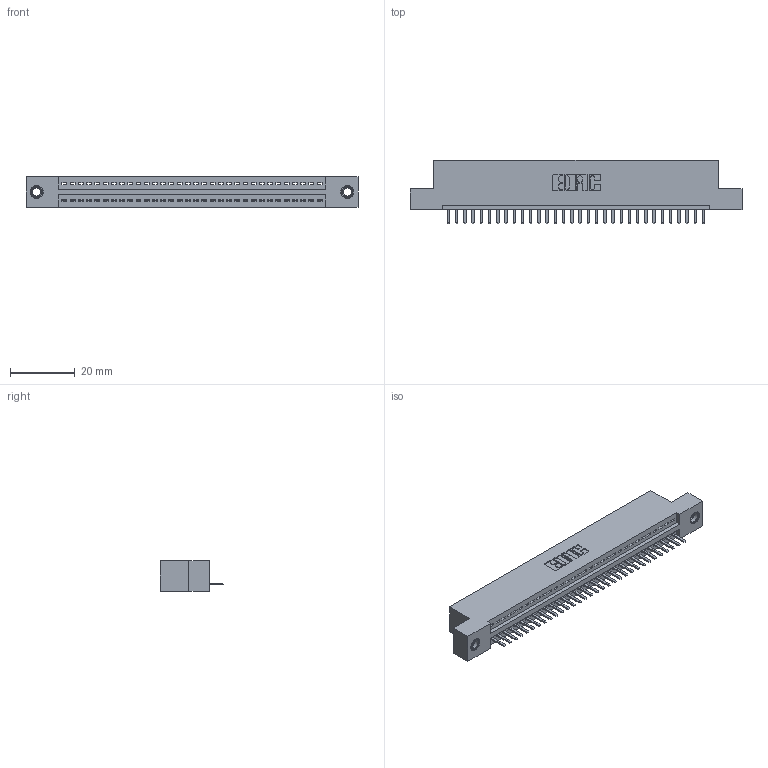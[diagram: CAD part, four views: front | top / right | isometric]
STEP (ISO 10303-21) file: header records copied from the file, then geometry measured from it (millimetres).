
FILE_DESCRIPTION (( 'STEP AP203' ), '1' );
FILE_NAME ('395-032-520-107.STEP', '2019-10-19T13:41:24', ( '' ), ( '' ), 'SwSTEP 2.0', 'SolidWorks 2016', '' );
FILE_SCHEMA (( 'CONFIG_CONTROL_DESIGN' ));
Length unit declared in the file: inch
Products named in the file (4): 345-250-001_345-250-005-103; 345 Part_Flush Mounting Lugs - 0.156 Dia-TI; 345-292-001_345-293-120; 395-032-520-107
Assembly tree (35 placements, depth 2):
  395-032-520-107
    345 Part_Flush Mounting Lugs - 0.156 Dia-TI
    345-292-001_345-293-120  x32
    345-250-001_345-250-005-103  x2
Bounding box: 102.49 x 19.68 x 9.4 mm (x, y, z)
Volume: 9547 mm3; surface area: 12282.7 mm2
Topology: 35 solids, 35 shells, 2170 faces, 6365 edges, 4150 vertices
Faces by surface type: plane 1456, cylinder 698, cone 12, torus 4
Entity records: 26730 total; most frequent: CARTESIAN_POINT 4623, ORIENTED_EDGE 4570, DIRECTION 4067, EDGE_CURVE 2285, LINE 2001, VECTOR 2001, VERTEX_POINT 1516, AXIS2_PLACEMENT_3D 1033
